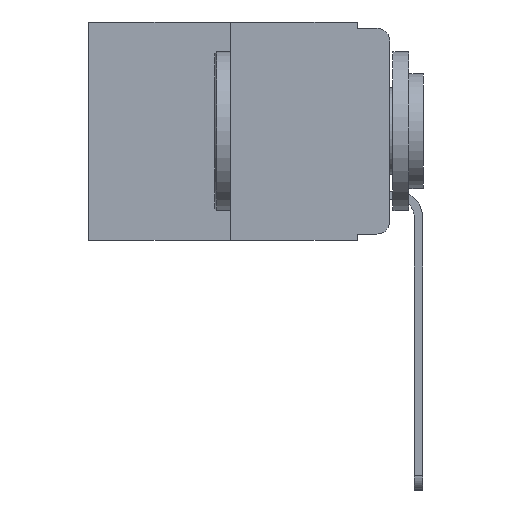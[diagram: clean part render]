
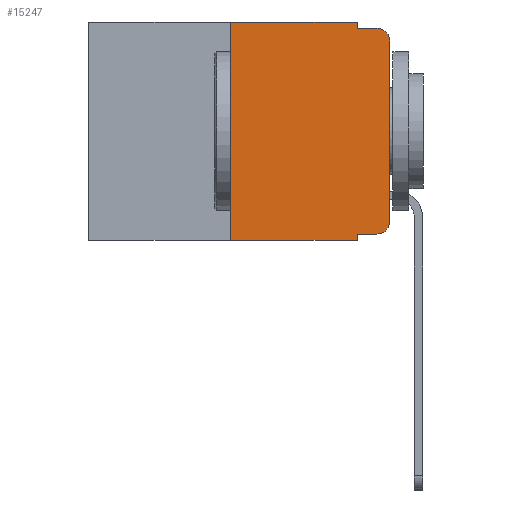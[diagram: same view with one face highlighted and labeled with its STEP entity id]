
A CAD part, left-side view. The second image highlights one B-rep face of the part: STEP entity #15247.
In plain terms, the highlighted planar face has unit normal (-1, 0, 0).
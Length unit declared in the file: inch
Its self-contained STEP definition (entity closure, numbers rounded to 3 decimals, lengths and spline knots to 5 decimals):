
#78 = DIRECTION ( 'NONE',  ( 0., -1., 0. ) ) ;
#139 = EDGE_CURVE ( 'NONE', #13174, #4434, #2605, .T. ) ;
#270 = CARTESIAN_POINT ( 'NONE',  ( 0., 0.473, 0. ) ) ;
#762 = DIRECTION ( 'NONE',  ( 0., -1., 0. ) ) ;
#809 = DIRECTION ( 'NONE',  ( 0., 0., 1. ) ) ;
#884 = CARTESIAN_POINT ( 'NONE',  ( 0., 0.051, -0.01 ) ) ;
#1171 = ORIENTED_EDGE ( 'NONE', *, *, #4367, .T. ) ;
#1533 = LINE ( 'NONE', #7326, #11342 ) ;
#1597 = DIRECTION ( 'NONE',  ( 0., 0., -1. ) ) ;
#1814 = VERTEX_POINT ( 'NONE', #10254 ) ;
#2162 = CARTESIAN_POINT ( 'NONE',  ( 0., 0.051, -0.343 ) ) ;
#2289 = VERTEX_POINT ( 'NONE', #9848 ) ;
#2605 = LINE ( 'NONE', #7583, #15045 ) ;
#2616 = DIRECTION ( 'NONE',  ( 1., 0., 0. ) ) ;
#2922 = DIRECTION ( 'NONE',  ( 0., -1., 0. ) ) ;
#3055 = AXIS2_PLACEMENT_3D ( 'NONE', #270, #2616, #6509 ) ;
#3128 = ORIENTED_EDGE ( 'NONE', *, *, #15834, .F. ) ;
#3439 = ORIENTED_EDGE ( 'NONE', *, *, #139, .F. ) ;
#3626 = ORIENTED_EDGE ( 'NONE', *, *, #9311, .T. ) ;
#3743 = EDGE_LOOP ( 'NONE', ( #3626, #6630, #12390, #3128, #14465, #3439, #14526, #13925, #1171, #4273 ) ) ;
#3845 = VECTOR ( 'NONE', #8404, 39.37008 ) ;
#3902 = LINE ( 'NONE', #6804, #16378 ) ;
#3983 = CARTESIAN_POINT ( 'NONE',  ( 0., 0.051, -0.333 ) ) ;
#4190 = EDGE_CURVE ( 'NONE', #1814, #2289, #8609, .T. ) ;
#4273 = ORIENTED_EDGE ( 'NONE', *, *, #4514, .T. ) ;
#4305 = DIRECTION ( 'NONE',  ( -1., 0., 0. ) ) ;
#4356 = DIRECTION ( 'NONE',  ( 0., 0., -1. ) ) ;
#4367 = EDGE_CURVE ( 'NONE', #10874, #12153, #15489, .T. ) ;
#4412 = VECTOR ( 'NONE', #15051, 39.37008 ) ;
#4434 = VERTEX_POINT ( 'NONE', #6489 ) ;
#4514 = EDGE_CURVE ( 'NONE', #12153, #16390, #15064, .T. ) ;
#4595 = EDGE_CURVE ( 'NONE', #4434, #12734, #5187, .T. ) ;
#5187 = LINE ( 'NONE', #5687, #10622 ) ;
#5564 = DIRECTION ( 'NONE',  ( 0., 0., -1. ) ) ;
#5587 = CARTESIAN_POINT ( 'NONE',  ( 0., 0.25, -0.343 ) ) ;
#5687 = CARTESIAN_POINT ( 'NONE',  ( 0., 0.473, 0. ) ) ;
#6275 = EDGE_CURVE ( 'NONE', #10530, #2289, #7316, .T. ) ;
#6489 = CARTESIAN_POINT ( 'NONE',  ( 0., 0.25, 0. ) ) ;
#6509 = DIRECTION ( 'NONE',  ( 0., 0., -1. ) ) ;
#6630 = ORIENTED_EDGE ( 'NONE', *, *, #6275, .T. ) ;
#6804 = CARTESIAN_POINT ( 'NONE',  ( 0., 0.051, 0. ) ) ;
#7316 = CIRCLE ( 'NONE', #16293, 0.02 ) ;
#7326 = CARTESIAN_POINT ( 'NONE',  ( 0., 0., 0. ) ) ;
#7583 = CARTESIAN_POINT ( 'NONE',  ( 0., 0.25, 0. ) ) ;
#7703 = LINE ( 'NONE', #15452, #11154 ) ;
#8091 = CARTESIAN_POINT ( 'NONE',  ( 0., 0.02, -0.03 ) ) ;
#8105 = EDGE_CURVE ( 'NONE', #13174, #8187, #7703, .T. ) ;
#8187 = VERTEX_POINT ( 'NONE', #2162 ) ;
#8404 = DIRECTION ( 'NONE',  ( 0., 0., -1. ) ) ;
#8609 = LINE ( 'NONE', #884, #4412 ) ;
#9311 = EDGE_CURVE ( 'NONE', #16390, #10530, #1533, .T. ) ;
#9517 = CARTESIAN_POINT ( 'NONE',  ( 0., 0.02, -0.333 ) ) ;
#9762 = EDGE_CURVE ( 'NONE', #10874, #8187, #3902, .T. ) ;
#9848 = CARTESIAN_POINT ( 'NONE',  ( 0., 0.02, -0.01 ) ) ;
#9892 = DIRECTION ( 'NONE',  ( 0., 0., 1. ) ) ;
#10254 = CARTESIAN_POINT ( 'NONE',  ( 0., 0.051, -0.01 ) ) ;
#10392 = PLANE ( 'NONE',  #3055 ) ;
#10530 = VERTEX_POINT ( 'NONE', #16074 ) ;
#10622 = VECTOR ( 'NONE', #762, 39.37008 ) ;
#10677 = LINE ( 'NONE', #16089, #3845 ) ;
#10874 = VERTEX_POINT ( 'NONE', #3983 ) ;
#11154 = VECTOR ( 'NONE', #78, 39.37008 ) ;
#11342 = VECTOR ( 'NONE', #9892, 39.37008 ) ;
#12076 = DIRECTION ( 'NONE',  ( -1., 0., 0. ) ) ;
#12153 = VERTEX_POINT ( 'NONE', #9517 ) ;
#12390 = ORIENTED_EDGE ( 'NONE', *, *, #4190, .F. ) ;
#12613 = FACE_OUTER_BOUND ( 'NONE', #3743, .T. ) ;
#12734 = VERTEX_POINT ( 'NONE', #13892 ) ;
#13174 = VERTEX_POINT ( 'NONE', #5587 ) ;
#13279 = CARTESIAN_POINT ( 'NONE',  ( 0., 0., -0.313 ) ) ;
#13377 = CARTESIAN_POINT ( 'NONE',  ( 0., 0.02, -0.313 ) ) ;
#13892 = CARTESIAN_POINT ( 'NONE',  ( 0., 0.051, 0. ) ) ;
#13925 = ORIENTED_EDGE ( 'NONE', *, *, #9762, .F. ) ;
#14465 = ORIENTED_EDGE ( 'NONE', *, *, #4595, .F. ) ;
#14526 = ORIENTED_EDGE ( 'NONE', *, *, #8105, .T. ) ;
#15045 = VECTOR ( 'NONE', #809, 39.37008 ) ;
#15051 = DIRECTION ( 'NONE',  ( 0., -1., 0. ) ) ;
#15064 = CIRCLE ( 'NONE', #16659, 0.02 ) ;
#15247 = ADVANCED_FACE ( 'NONE', ( #12613 ), #10392, .F. ) ;
#15401 = CARTESIAN_POINT ( 'NONE',  ( 0., 0.051, -0.333 ) ) ;
#15452 = CARTESIAN_POINT ( 'NONE',  ( 0., 0.473, -0.343 ) ) ;
#15489 = LINE ( 'NONE', #15401, #16281 ) ;
#15834 = EDGE_CURVE ( 'NONE', #12734, #1814, #10677, .T. ) ;
#16074 = CARTESIAN_POINT ( 'NONE',  ( 0., 0., -0.03 ) ) ;
#16089 = CARTESIAN_POINT ( 'NONE',  ( 0., 0.051, 0. ) ) ;
#16281 = VECTOR ( 'NONE', #2922, 39.37008 ) ;
#16293 = AXIS2_PLACEMENT_3D ( 'NONE', #8091, #4305, #1597 ) ;
#16378 = VECTOR ( 'NONE', #5564, 39.37008 ) ;
#16390 = VERTEX_POINT ( 'NONE', #13279 ) ;
#16659 = AXIS2_PLACEMENT_3D ( 'NONE', #13377, #12076, #4356 ) ;
